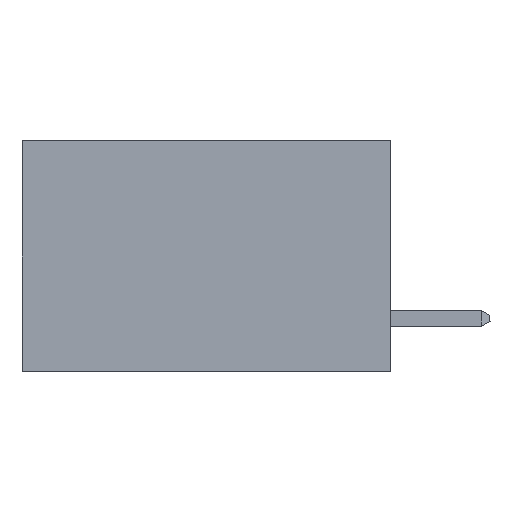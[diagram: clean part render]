
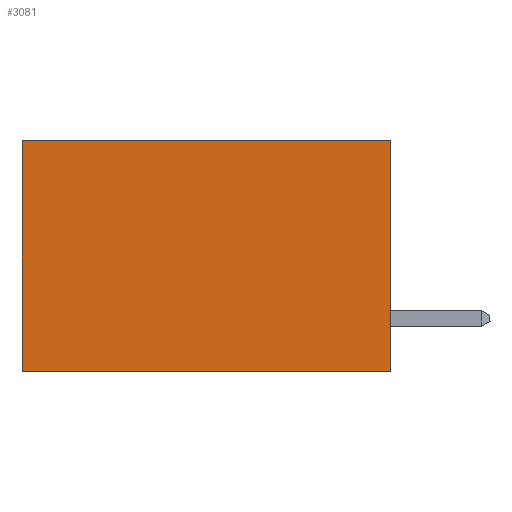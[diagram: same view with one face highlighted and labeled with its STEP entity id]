
A CAD part, left-side view. The second image highlights one B-rep face of the part: STEP entity #3081.
In plain terms, the highlighted planar face has unit normal (-1, 0, 0).
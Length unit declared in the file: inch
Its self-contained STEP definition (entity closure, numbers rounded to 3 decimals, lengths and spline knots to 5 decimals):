
#268 = VECTOR ( 'NONE', #676, 39.37008 ) ;
#347 = VECTOR ( 'NONE', #19857, 39.37008 ) ;
#676 = DIRECTION ( 'NONE',  ( 0., 1., 0. ) ) ;
#937 = LINE ( 'NONE', #20081, #347 ) ;
#1382 = ORIENTED_EDGE ( 'NONE', *, *, #4875, .F. ) ;
#1616 = LINE ( 'NONE', #20869, #11310 ) ;
#2445 = FACE_OUTER_BOUND ( 'NONE', #6181, .T. ) ;
#3081 = ADVANCED_FACE ( 'NONE', ( #2445 ), #5092, .F. ) ;
#3736 = VECTOR ( 'NONE', #7419, 39.37008 ) ;
#4297 = LINE ( 'NONE', #7078, #3736 ) ;
#4875 = EDGE_CURVE ( 'NONE', #6399, #14089, #937, .T. ) ;
#5092 = PLANE ( 'NONE',  #10795 ) ;
#6181 = EDGE_LOOP ( 'NONE', ( #14747, #1382, #6267, #16415 ) ) ;
#6267 = ORIENTED_EDGE ( 'NONE', *, *, #7105, .F. ) ;
#6399 = VERTEX_POINT ( 'NONE', #23133 ) ;
#6649 = VERTEX_POINT ( 'NONE', #16143 ) ;
#6839 = CARTESIAN_POINT ( 'NONE',  ( 0.277, 0., 0. ) ) ;
#7078 = CARTESIAN_POINT ( 'NONE',  ( 0.277, 0., -0.37 ) ) ;
#7105 = EDGE_CURVE ( 'NONE', #13130, #6399, #4297, .T. ) ;
#7419 = DIRECTION ( 'NONE',  ( 0., 0., -1. ) ) ;
#9837 = CARTESIAN_POINT ( 'NONE',  ( 0.277, 0., 0. ) ) ;
#10033 = LINE ( 'NONE', #9837, #268 ) ;
#10159 = DIRECTION ( 'NONE',  ( 0., 0., -1. ) ) ;
#10795 = AXIS2_PLACEMENT_3D ( 'NONE', #12910, #12746, #13894 ) ;
#11310 = VECTOR ( 'NONE', #10159, 39.37008 ) ;
#12201 = EDGE_CURVE ( 'NONE', #13130, #6649, #10033, .T. ) ;
#12746 = DIRECTION ( 'NONE',  ( 1., 0., 0. ) ) ;
#12910 = CARTESIAN_POINT ( 'NONE',  ( 0.277, 0., -0.37 ) ) ;
#13130 = VERTEX_POINT ( 'NONE', #6839 ) ;
#13894 = DIRECTION ( 'NONE',  ( 0., 0., -1. ) ) ;
#14089 = VERTEX_POINT ( 'NONE', #14937 ) ;
#14747 = ORIENTED_EDGE ( 'NONE', *, *, #15934, .T. ) ;
#14937 = CARTESIAN_POINT ( 'NONE',  ( 0.277, 0.59, -0.37 ) ) ;
#15934 = EDGE_CURVE ( 'NONE', #6649, #14089, #1616, .T. ) ;
#16143 = CARTESIAN_POINT ( 'NONE',  ( 0.277, 0.59, 0. ) ) ;
#16415 = ORIENTED_EDGE ( 'NONE', *, *, #12201, .T. ) ;
#19857 = DIRECTION ( 'NONE',  ( 0., 1., 0. ) ) ;
#20081 = CARTESIAN_POINT ( 'NONE',  ( 0.277, 0., -0.37 ) ) ;
#20869 = CARTESIAN_POINT ( 'NONE',  ( 0.277, 0.59, -0.37 ) ) ;
#23133 = CARTESIAN_POINT ( 'NONE',  ( 0.277, 0., -0.37 ) ) ;
